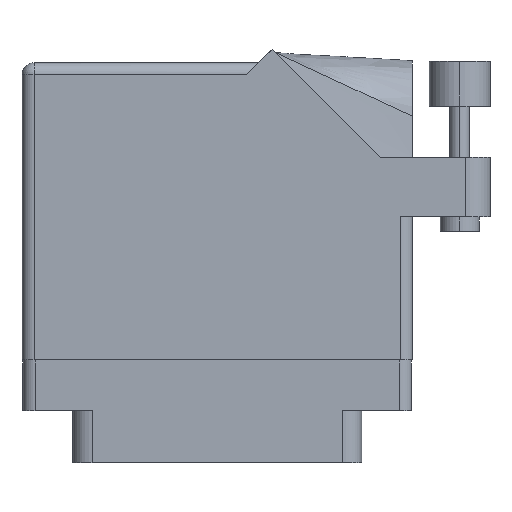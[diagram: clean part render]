
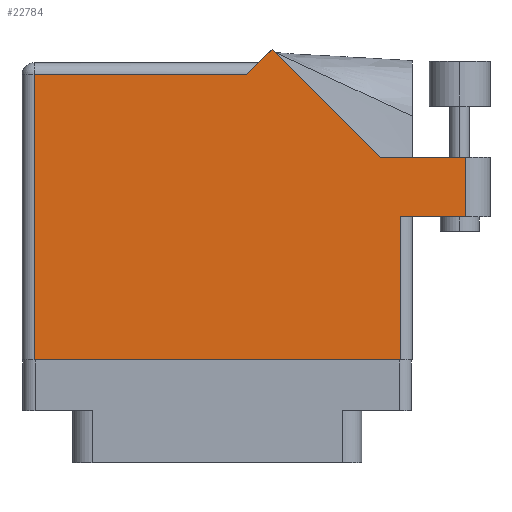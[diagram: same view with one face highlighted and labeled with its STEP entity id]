
A CAD part, front view. The second image highlights one B-rep face of the part: STEP entity #22784.
In plain terms, the highlighted face is planar.
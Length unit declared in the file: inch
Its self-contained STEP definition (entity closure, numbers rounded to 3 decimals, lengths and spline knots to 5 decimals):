
#150 = VERTEX_POINT ( 'NONE', #11189 ) ;
#310 = DIRECTION ( 'NONE',  ( 0., 1., 0. ) ) ;
#401 = VECTOR ( 'NONE', #665, 39.37008 ) ;
#665 = DIRECTION ( 'NONE',  ( 1., 0., 0. ) ) ;
#1952 = VECTOR ( 'NONE', #310, 39.37008 ) ;
#2416 = CARTESIAN_POINT ( 'NONE',  ( 2.285, 0.737, 0. ) ) ;
#3248 = CARTESIAN_POINT ( 'NONE',  ( 0., 0., 0. ) ) ;
#3302 = EDGE_CURVE ( 'NONE', #10479, #150, #12813, .T. ) ;
#3728 = VECTOR ( 'NONE', #21922, 39.37008 ) ;
#3950 = VECTOR ( 'NONE', #8483, 39.37008 ) ;
#4136 = VECTOR ( 'NONE', #26924, 39.37008 ) ;
#4545 = FACE_OUTER_BOUND ( 'NONE', #21328, .T. ) ;
#4737 = CARTESIAN_POINT ( 'NONE',  ( 2.285, 1.044, 0. ) ) ;
#4868 = DIRECTION ( 'NONE',  ( -1., 0., 0. ) ) ;
#5615 = EDGE_CURVE ( 'NONE', #27864, #23443, #9592, .T. ) ;
#5752 = CARTESIAN_POINT ( 'NONE',  ( 0., 1.468, 0. ) ) ;
#6340 = LINE ( 'NONE', #28739, #19864 ) ;
#6929 = VECTOR ( 'NONE', #24324, 39.37008 ) ;
#7928 = CARTESIAN_POINT ( 'NONE',  ( 1.948, 0.737, 0. ) ) ;
#7972 = CARTESIAN_POINT ( 'NONE',  ( 1.948, 0.737, 0. ) ) ;
#8483 = DIRECTION ( 'NONE',  ( -1., 0., 0. ) ) ;
#9240 = LINE ( 'NONE', #3248, #401 ) ;
#9368 = CARTESIAN_POINT ( 'NONE',  ( 1.217, 1.53, 0. ) ) ;
#9592 = LINE ( 'NONE', #7972, #1952 ) ;
#9652 = LINE ( 'NONE', #9368, #16371 ) ;
#9732 = EDGE_CURVE ( 'NONE', #23443, #17765, #6340, .T. ) ;
#10479 = VERTEX_POINT ( 'NONE', #20884 ) ;
#11138 = EDGE_CURVE ( 'NONE', #33735, #31166, #18043, .T. ) ;
#11189 = CARTESIAN_POINT ( 'NONE',  ( 0.062, 1.468, 0. ) ) ;
#12813 = LINE ( 'NONE', #5752, #3950 ) ;
#13023 = DIRECTION ( 'NONE',  ( 0., 0., -1. ) ) ;
#14112 = VERTEX_POINT ( 'NONE', #34386 ) ;
#15707 = CARTESIAN_POINT ( 'NONE',  ( 2.41, 1.044, 0. ) ) ;
#16073 = EDGE_CURVE ( 'NONE', #17765, #33735, #19595, .T. ) ;
#16371 = VECTOR ( 'NONE', #28682, 39.37008 ) ;
#16611 = ORIENTED_EDGE ( 'NONE', *, *, #30241, .T. ) ;
#17765 = VERTEX_POINT ( 'NONE', #2416 ) ;
#17959 = PLANE ( 'NONE',  #23469 ) ;
#18043 = LINE ( 'NONE', #15707, #3728 ) ;
#19595 = LINE ( 'NONE', #4737, #6929 ) ;
#19864 = VECTOR ( 'NONE', #30977, 39.37008 ) ;
#20884 = CARTESIAN_POINT ( 'NONE',  ( 1.155, 1.468, 0. ) ) ;
#21328 = EDGE_LOOP ( 'NONE', ( #28051, #25310, #24795, #16611, #29025, #21960, #30013, #34724, #25812 ) ) ;
#21922 = DIRECTION ( 'NONE',  ( -1., 0., 0. ) ) ;
#21957 = EDGE_CURVE ( 'NONE', #14112, #27864, #9240, .T. ) ;
#21960 = ORIENTED_EDGE ( 'NONE', *, *, #3302, .T. ) ;
#22784 = ADVANCED_FACE ( 'NONE', ( #4545 ), #17959, .F. ) ;
#23443 = VERTEX_POINT ( 'NONE', #7928 ) ;
#23469 = AXIS2_PLACEMENT_3D ( 'NONE', #31627, #13023, #4868 ) ;
#24324 = DIRECTION ( 'NONE',  ( 0., 1., 0. ) ) ;
#24480 = CARTESIAN_POINT ( 'NONE',  ( 0.062, 0., 0. ) ) ;
#24567 = CARTESIAN_POINT ( 'NONE',  ( 1.84442, 1.044, 0. ) ) ;
#24795 = ORIENTED_EDGE ( 'NONE', *, *, #11138, .T. ) ;
#25310 = ORIENTED_EDGE ( 'NONE', *, *, #16073, .T. ) ;
#25812 = ORIENTED_EDGE ( 'NONE', *, *, #5615, .T. ) ;
#26924 = DIRECTION ( 'NONE',  ( -0.707, 0.707, 0. ) ) ;
#27535 = VERTEX_POINT ( 'NONE', #29277 ) ;
#27864 = VERTEX_POINT ( 'NONE', #31540 ) ;
#28051 = ORIENTED_EDGE ( 'NONE', *, *, #9732, .T. ) ;
#28682 = DIRECTION ( 'NONE',  ( -0.707, -0.707, 0. ) ) ;
#28739 = CARTESIAN_POINT ( 'NONE',  ( 2.01, 0.737, 0. ) ) ;
#29025 = ORIENTED_EDGE ( 'NONE', *, *, #30774, .T. ) ;
#29277 = CARTESIAN_POINT ( 'NONE',  ( 1.28771, 1.60071, 0. ) ) ;
#29727 = EDGE_CURVE ( 'NONE', #150, #14112, #30293, .T. ) ;
#30013 = ORIENTED_EDGE ( 'NONE', *, *, #29727, .T. ) ;
#30241 = EDGE_CURVE ( 'NONE', #31166, #27535, #32813, .T. ) ;
#30293 = LINE ( 'NONE', #24480, #33269 ) ;
#30333 = DIRECTION ( 'NONE',  ( 0., -1., 0. ) ) ;
#30632 = CARTESIAN_POINT ( 'NONE',  ( 1.84442, 1.044, 0. ) ) ;
#30774 = EDGE_CURVE ( 'NONE', #27535, #10479, #9652, .T. ) ;
#30977 = DIRECTION ( 'NONE',  ( 1., 0., 0. ) ) ;
#31064 = CARTESIAN_POINT ( 'NONE',  ( 2.285, 1.044, 0. ) ) ;
#31166 = VERTEX_POINT ( 'NONE', #30632 ) ;
#31540 = CARTESIAN_POINT ( 'NONE',  ( 1.948, 0., 0. ) ) ;
#31627 = CARTESIAN_POINT ( 'NONE',  ( 0., 1.53, 0. ) ) ;
#32813 = LINE ( 'NONE', #24567, #4136 ) ;
#33269 = VECTOR ( 'NONE', #30333, 39.37008 ) ;
#33735 = VERTEX_POINT ( 'NONE', #31064 ) ;
#34386 = CARTESIAN_POINT ( 'NONE',  ( 0.062, 0., 0. ) ) ;
#34724 = ORIENTED_EDGE ( 'NONE', *, *, #21957, .T. ) ;
